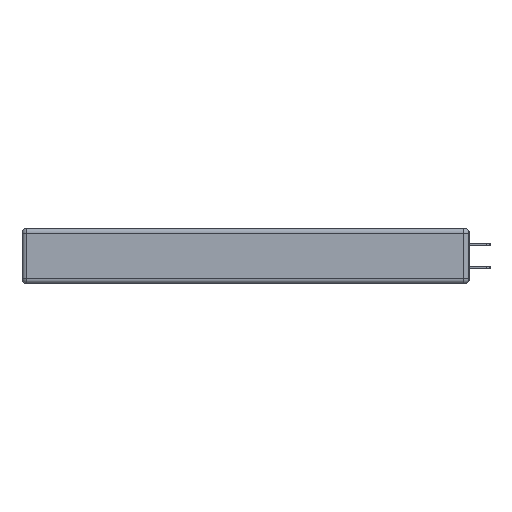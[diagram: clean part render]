
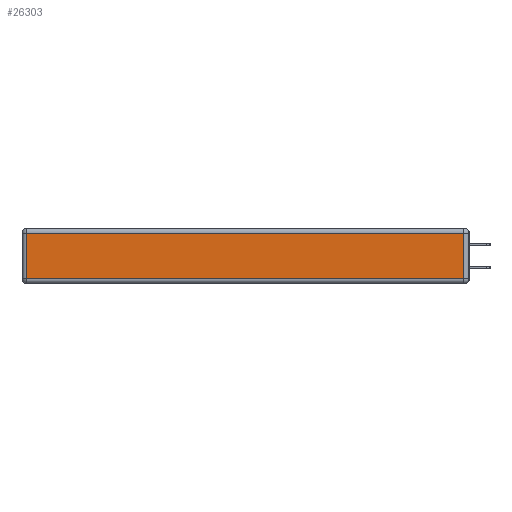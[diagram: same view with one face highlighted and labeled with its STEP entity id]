
A CAD part, left-side view. The second image highlights one B-rep face of the part: STEP entity #26303.
In plain terms, the highlighted planar face has unit normal (-1, 0, 0).
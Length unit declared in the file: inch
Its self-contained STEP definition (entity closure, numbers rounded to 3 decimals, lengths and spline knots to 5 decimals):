
#227 = EDGE_CURVE ( 'NONE', #25928, #9998, #19767, .T. ) ;
#1416 = DIRECTION ( 'NONE',  ( 0., 1., 0. ) ) ;
#1710 = CARTESIAN_POINT ( 'NONE',  ( 0., 2.75, -0.03 ) ) ;
#2969 = DIRECTION ( 'NONE',  ( 0., 0., 1. ) ) ;
#4375 = EDGE_CURVE ( 'NONE', #6973, #7984, #7962, .T. ) ;
#5135 = PLANE ( 'NONE',  #6076 ) ;
#5238 = CARTESIAN_POINT ( 'NONE',  ( 0., 0., -0.343 ) ) ;
#6076 = AXIS2_PLACEMENT_3D ( 'NONE', #5238, #27579, #2969 ) ;
#6879 = DIRECTION ( 'NONE',  ( 0., -1., 0. ) ) ;
#6973 = VERTEX_POINT ( 'NONE', #27512 ) ;
#7293 = VECTOR ( 'NONE', #1416, 39.37008 ) ;
#7962 = LINE ( 'NONE', #18980, #8680 ) ;
#7984 = VERTEX_POINT ( 'NONE', #18131 ) ;
#8508 = DIRECTION ( 'NONE',  ( 0., 0., 1. ) ) ;
#8680 = VECTOR ( 'NONE', #9659, 39.37008 ) ;
#9261 = EDGE_CURVE ( 'NONE', #9998, #6973, #27914, .T. ) ;
#9659 = DIRECTION ( 'NONE',  ( 0., 0., -1. ) ) ;
#9998 = VERTEX_POINT ( 'NONE', #18139 ) ;
#10360 = ORIENTED_EDGE ( 'NONE', *, *, #12452, .T. ) ;
#11528 = ORIENTED_EDGE ( 'NONE', *, *, #4375, .T. ) ;
#11839 = LINE ( 'NONE', #23391, #20250 ) ;
#12452 = EDGE_CURVE ( 'NONE', #7984, #25928, #11839, .T. ) ;
#16860 = CARTESIAN_POINT ( 'NONE',  ( 0., 0.03, -0.313 ) ) ;
#18131 = CARTESIAN_POINT ( 'NONE',  ( 0., 2.72, -0.313 ) ) ;
#18139 = CARTESIAN_POINT ( 'NONE',  ( 0., 0.03, -0.03 ) ) ;
#18980 = CARTESIAN_POINT ( 'NONE',  ( 0., 2.72, -0.343 ) ) ;
#19767 = LINE ( 'NONE', #28530, #26052 ) ;
#20250 = VECTOR ( 'NONE', #6879, 39.37008 ) ;
#20931 = ORIENTED_EDGE ( 'NONE', *, *, #9261, .T. ) ;
#23391 = CARTESIAN_POINT ( 'NONE',  ( 0., 0., -0.313 ) ) ;
#23889 = EDGE_LOOP ( 'NONE', ( #10360, #28158, #20931, #11528 ) ) ;
#24003 = FACE_OUTER_BOUND ( 'NONE', #23889, .T. ) ;
#25928 = VERTEX_POINT ( 'NONE', #16860 ) ;
#26052 = VECTOR ( 'NONE', #8508, 39.37008 ) ;
#26303 = ADVANCED_FACE ( 'NONE', ( #24003 ), #5135, .T. ) ;
#27512 = CARTESIAN_POINT ( 'NONE',  ( 0., 2.72, -0.03 ) ) ;
#27579 = DIRECTION ( 'NONE',  ( -1., 0., 0. ) ) ;
#27914 = LINE ( 'NONE', #1710, #7293 ) ;
#28158 = ORIENTED_EDGE ( 'NONE', *, *, #227, .T. ) ;
#28530 = CARTESIAN_POINT ( 'NONE',  ( 0., 0.03, -0.343 ) ) ;
